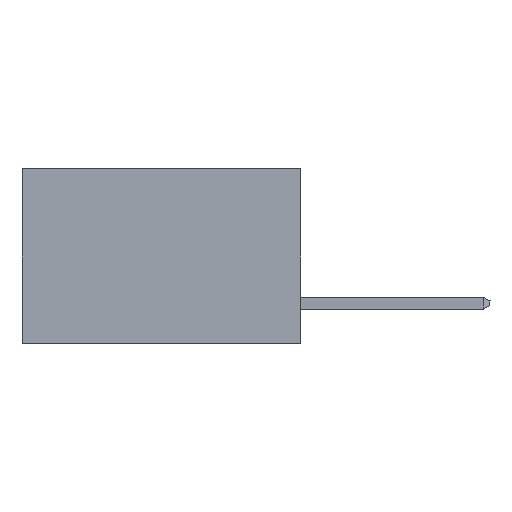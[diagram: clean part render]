
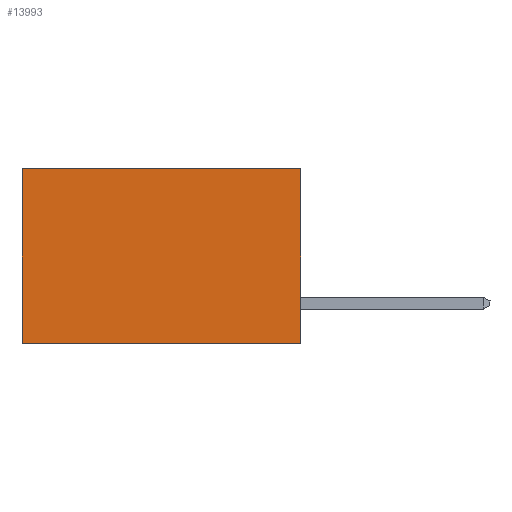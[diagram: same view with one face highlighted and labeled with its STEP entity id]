
A CAD part, left-side view. The second image highlights one B-rep face of the part: STEP entity #13993.
In plain terms, the highlighted planar face has unit normal (-1, 0, 0).
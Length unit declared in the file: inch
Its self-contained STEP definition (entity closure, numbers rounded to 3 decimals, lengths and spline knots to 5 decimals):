
#96 = DIRECTION ( 'NONE',  ( 0., 0., -1. ) ) ;
#251 = CARTESIAN_POINT ( 'NONE',  ( 0.277, 0., -0.37 ) ) ;
#736 = AXIS2_PLACEMENT_3D ( 'NONE', #5984, #7252, #16186 ) ;
#831 = EDGE_LOOP ( 'NONE', ( #1792, #3449, #5692, #3867 ) ) ;
#1106 = EDGE_CURVE ( 'NONE', #4109, #6611, #11209, .T. ) ;
#1676 = CARTESIAN_POINT ( 'NONE',  ( 0.277, 0.59, -0.37 ) ) ;
#1740 = VECTOR ( 'NONE', #6736, 39.37008 ) ;
#1792 = ORIENTED_EDGE ( 'NONE', *, *, #10567, .T. ) ;
#1811 = DIRECTION ( 'NONE',  ( 0., 0., -1. ) ) ;
#2139 = CARTESIAN_POINT ( 'NONE',  ( 0.277, 0.59, 0. ) ) ;
#2371 = CARTESIAN_POINT ( 'NONE',  ( 0.277, 0., 0. ) ) ;
#3449 = ORIENTED_EDGE ( 'NONE', *, *, #16238, .F. ) ;
#3867 = ORIENTED_EDGE ( 'NONE', *, *, #1106, .T. ) ;
#4109 = VERTEX_POINT ( 'NONE', #2371 ) ;
#4714 = VECTOR ( 'NONE', #96, 39.37008 ) ;
#4845 = CARTESIAN_POINT ( 'NONE',  ( 0.277, 0., 0. ) ) ;
#5692 = ORIENTED_EDGE ( 'NONE', *, *, #12986, .F. ) ;
#5984 = CARTESIAN_POINT ( 'NONE',  ( 0.277, 0., -0.37 ) ) ;
#6611 = VERTEX_POINT ( 'NONE', #2139 ) ;
#6736 = DIRECTION ( 'NONE',  ( 0., 1., 0. ) ) ;
#7252 = DIRECTION ( 'NONE',  ( 1., 0., 0. ) ) ;
#8106 = VECTOR ( 'NONE', #8849, 39.37008 ) ;
#8234 = LINE ( 'NONE', #1676, #8671 ) ;
#8671 = VECTOR ( 'NONE', #1811, 39.37008 ) ;
#8849 = DIRECTION ( 'NONE',  ( 0., 1., 0. ) ) ;
#8936 = CARTESIAN_POINT ( 'NONE',  ( 0.277, 0., -0.37 ) ) ;
#9376 = VERTEX_POINT ( 'NONE', #10488 ) ;
#10473 = CARTESIAN_POINT ( 'NONE',  ( 0.277, 0., -0.37 ) ) ;
#10488 = CARTESIAN_POINT ( 'NONE',  ( 0.277, 0.59, -0.37 ) ) ;
#10567 = EDGE_CURVE ( 'NONE', #6611, #9376, #8234, .T. ) ;
#11209 = LINE ( 'NONE', #4845, #8106 ) ;
#11610 = LINE ( 'NONE', #10473, #4714 ) ;
#12144 = LINE ( 'NONE', #251, #1740 ) ;
#12986 = EDGE_CURVE ( 'NONE', #4109, #15417, #11610, .T. ) ;
#13790 = PLANE ( 'NONE',  #736 ) ;
#13993 = ADVANCED_FACE ( 'NONE', ( #15872 ), #13790, .F. ) ;
#15417 = VERTEX_POINT ( 'NONE', #8936 ) ;
#15872 = FACE_OUTER_BOUND ( 'NONE', #831, .T. ) ;
#16186 = DIRECTION ( 'NONE',  ( 0., 0., -1. ) ) ;
#16238 = EDGE_CURVE ( 'NONE', #15417, #9376, #12144, .T. ) ;
